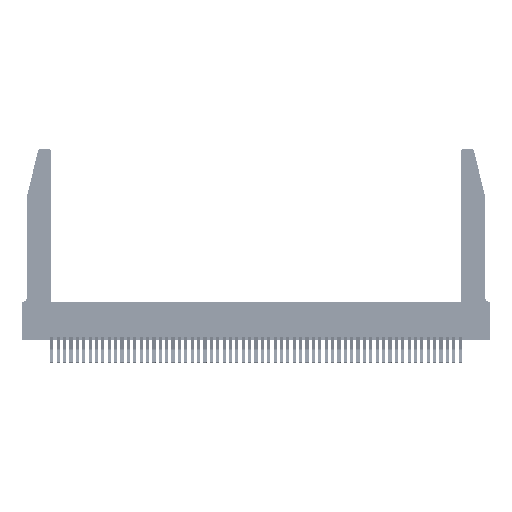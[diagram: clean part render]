
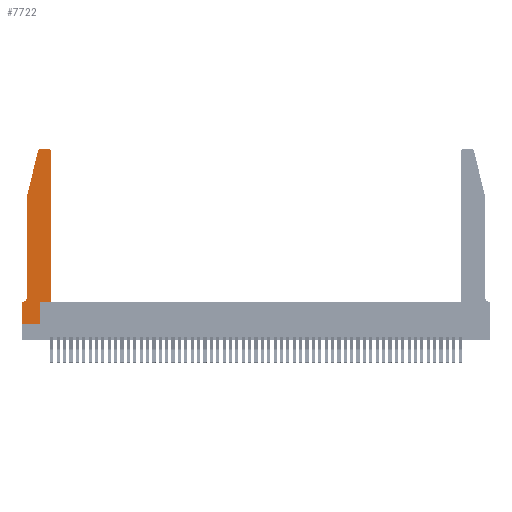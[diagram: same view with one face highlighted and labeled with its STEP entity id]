
A CAD part, top view. The second image highlights one B-rep face of the part: STEP entity #7722.
In plain terms, the highlighted planar face has unit normal (0, 0, 1).
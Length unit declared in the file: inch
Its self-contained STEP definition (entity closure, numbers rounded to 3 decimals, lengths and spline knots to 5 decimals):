
#462 = VERTEX_POINT ( 'NONE', #19016 ) ;
#1192 = VECTOR ( 'NONE', #32694, 39.37008 ) ;
#2263 = CIRCLE ( 'NONE', #45965, 0.03 ) ;
#2456 = VECTOR ( 'NONE', #37878, 39.37008 ) ;
#2739 = DIRECTION ( 'NONE',  ( 0., -1., 0. ) ) ;
#3266 = CARTESIAN_POINT ( 'NONE',  ( 0., 0., 0.37 ) ) ;
#3634 = EDGE_CURVE ( 'NONE', #33077, #462, #50777, .T. ) ;
#3919 = AXIS2_PLACEMENT_3D ( 'NONE', #16741, #32958, #40990 ) ;
#3988 = CARTESIAN_POINT ( 'NONE',  ( 0.0755, 0.35, 0.37 ) ) ;
#4423 = CARTESIAN_POINT ( 'NONE',  ( 0.25487, 2.72718, 0.37 ) ) ;
#4983 = LINE ( 'NONE', #38962, #16243 ) ;
#5503 = EDGE_CURVE ( 'NONE', #47868, #22579, #41599, .T. ) ;
#5510 = ORIENTED_EDGE ( 'NONE', *, *, #7617, .T. ) ;
#6280 = DIRECTION ( 'NONE',  ( 1., 0., 0. ) ) ;
#6669 = CARTESIAN_POINT ( 'NONE',  ( 0., 0.35, 0.37 ) ) ;
#7617 = EDGE_CURVE ( 'NONE', #16330, #10498, #29271, .T. ) ;
#7619 = DIRECTION ( 'NONE',  ( 0., -1., 0. ) ) ;
#7722 = ADVANCED_FACE ( 'NONE', ( #21538 ), #30600, .T. ) ;
#7946 = DIRECTION ( 'NONE',  ( 0., 0., 1. ) ) ;
#8790 = ORIENTED_EDGE ( 'NONE', *, *, #37576, .T. ) ;
#9179 = EDGE_CURVE ( 'NONE', #462, #36047, #2263, .T. ) ;
#9566 = VECTOR ( 'NONE', #16851, 39.37008 ) ;
#10246 = CARTESIAN_POINT ( 'NONE',  ( 0.0055, 0.35, 0.37 ) ) ;
#10498 = VERTEX_POINT ( 'NONE', #32687 ) ;
#10767 = ORIENTED_EDGE ( 'NONE', *, *, #16819, .T. ) ;
#11037 = VERTEX_POINT ( 'NONE', #47966 ) ;
#11060 = ORIENTED_EDGE ( 'NONE', *, *, #3634, .T. ) ;
#11523 = CARTESIAN_POINT ( 'NONE',  ( 0., 0.35, 0.37 ) ) ;
#12094 = EDGE_CURVE ( 'NONE', #36047, #35513, #42078, .T. ) ;
#12353 = EDGE_CURVE ( 'NONE', #41670, #31421, #33108, .T. ) ;
#12401 = ORIENTED_EDGE ( 'NONE', *, *, #9179, .T. ) ;
#12667 = AXIS2_PLACEMENT_3D ( 'NONE', #30721, #14342, #6280 ) ;
#12759 = CARTESIAN_POINT ( 'NONE',  ( 0.0755, 2., 0.37 ) ) ;
#12906 = CARTESIAN_POINT ( 'NONE',  ( 0.4505, 0.35, 0.37 ) ) ;
#14342 = DIRECTION ( 'NONE',  ( 0., 0., 1. ) ) ;
#14795 = ORIENTED_EDGE ( 'NONE', *, *, #12094, .T. ) ;
#16243 = VECTOR ( 'NONE', #31139, 39.37008 ) ;
#16330 = VERTEX_POINT ( 'NONE', #32920 ) ;
#16512 = DIRECTION ( 'NONE',  ( 1., 0., 0. ) ) ;
#16741 = CARTESIAN_POINT ( 'NONE',  ( 0.0055, 0.42, 0.37 ) ) ;
#16819 = EDGE_CURVE ( 'NONE', #31421, #20423, #24379, .T. ) ;
#16851 = DIRECTION ( 'NONE',  ( 1., 0., 0. ) ) ;
#16877 = DIRECTION ( 'NONE',  ( -0.239, -0.971, 0. ) ) ;
#17849 = ORIENTED_EDGE ( 'NONE', *, *, #46955, .T. ) ;
#18648 = DIRECTION ( 'NONE',  ( 1., 0., 0. ) ) ;
#19016 = CARTESIAN_POINT ( 'NONE',  ( 0.4505, 2.72, 0.37 ) ) ;
#19157 = DIRECTION ( 'NONE',  ( -1., 0., 0. ) ) ;
#19419 = CARTESIAN_POINT ( 'NONE',  ( 0.0755, 2., 0.37 ) ) ;
#20423 = VERTEX_POINT ( 'NONE', #3266 ) ;
#20910 = CIRCLE ( 'NONE', #3919, 0.07 ) ;
#21538 = FACE_OUTER_BOUND ( 'NONE', #23923, .T. ) ;
#21671 = LINE ( 'NONE', #19419, #48532 ) ;
#22579 = VERTEX_POINT ( 'NONE', #49021 ) ;
#22969 = CARTESIAN_POINT ( 'NONE',  ( 0.4505, 0.35, 0.37 ) ) ;
#23733 = ORIENTED_EDGE ( 'NONE', *, *, #28901, .T. ) ;
#23749 = VECTOR ( 'NONE', #2739, 39.37008 ) ;
#23923 = EDGE_LOOP ( 'NONE', ( #14795, #17849, #30488, #40120, #23733, #39189, #10767, #8790, #5510, #38531, #11060, #12401 ) ) ;
#24027 = DIRECTION ( 'NONE',  ( 0., 1., 0. ) ) ;
#24379 = LINE ( 'NONE', #47661, #23749 ) ;
#24537 = CARTESIAN_POINT ( 'NONE',  ( 0.4205, 2.72, 0.37 ) ) ;
#25027 = VECTOR ( 'NONE', #16877, 39.37008 ) ;
#26883 = CARTESIAN_POINT ( 'NONE',  ( 0.4205, 2.75, 0.37 ) ) ;
#28901 = EDGE_CURVE ( 'NONE', #11037, #41670, #20910, .T. ) ;
#29271 = LINE ( 'NONE', #34167, #2456 ) ;
#29872 = AXIS2_PLACEMENT_3D ( 'NONE', #6669, #30942, #18648 ) ;
#30488 = ORIENTED_EDGE ( 'NONE', *, *, #5503, .T. ) ;
#30600 = PLANE ( 'NONE',  #29872 ) ;
#30721 = CARTESIAN_POINT ( 'NONE',  ( 0.284, 2.72, 0.37 ) ) ;
#30942 = DIRECTION ( 'NONE',  ( 0., 0., 1. ) ) ;
#31139 = DIRECTION ( 'NONE',  ( 1., 0., 0. ) ) ;
#31213 = VECTOR ( 'NONE', #19157, 39.37008 ) ;
#31421 = VERTEX_POINT ( 'NONE', #11523 ) ;
#32687 = CARTESIAN_POINT ( 'NONE',  ( 0.2865, 0.35, 0.37 ) ) ;
#32694 = DIRECTION ( 'NONE',  ( -1., 0., 0. ) ) ;
#32920 = CARTESIAN_POINT ( 'NONE',  ( 0.2865, 0., 0.37 ) ) ;
#32958 = DIRECTION ( 'NONE',  ( 0., 0., -1. ) ) ;
#33077 = VERTEX_POINT ( 'NONE', #38055 ) ;
#33108 = LINE ( 'NONE', #3988, #1192 ) ;
#34167 = CARTESIAN_POINT ( 'NONE',  ( 0.2865, 0.35, 0.37 ) ) ;
#34839 = VECTOR ( 'NONE', #24027, 39.37008 ) ;
#35513 = VERTEX_POINT ( 'NONE', #43171 ) ;
#36047 = VERTEX_POINT ( 'NONE', #26883 ) ;
#37576 = EDGE_CURVE ( 'NONE', #20423, #16330, #4983, .T. ) ;
#37878 = DIRECTION ( 'NONE',  ( 0., 1., 0. ) ) ;
#38055 = CARTESIAN_POINT ( 'NONE',  ( 0.4505, 0.35, 0.37 ) ) ;
#38531 = ORIENTED_EDGE ( 'NONE', *, *, #48295, .T. ) ;
#38962 = CARTESIAN_POINT ( 'NONE',  ( 0., 0., 0.37 ) ) ;
#39189 = ORIENTED_EDGE ( 'NONE', *, *, #12353, .T. ) ;
#39619 = CIRCLE ( 'NONE', #12667, 0.03 ) ;
#40120 = ORIENTED_EDGE ( 'NONE', *, *, #47699, .T. ) ;
#40990 = DIRECTION ( 'NONE',  ( -1., 0., 0. ) ) ;
#41599 = LINE ( 'NONE', #12759, #25027 ) ;
#41670 = VERTEX_POINT ( 'NONE', #10246 ) ;
#42078 = LINE ( 'NONE', #43263, #31213 ) ;
#43171 = CARTESIAN_POINT ( 'NONE',  ( 0.284, 2.75, 0.37 ) ) ;
#43263 = CARTESIAN_POINT ( 'NONE',  ( 0.2605, 2.75, 0.37 ) ) ;
#45965 = AXIS2_PLACEMENT_3D ( 'NONE', #24537, #7946, #16512 ) ;
#46955 = EDGE_CURVE ( 'NONE', #35513, #47868, #39619, .T. ) ;
#47661 = CARTESIAN_POINT ( 'NONE',  ( 0., 0., 0.37 ) ) ;
#47699 = EDGE_CURVE ( 'NONE', #22579, #11037, #21671, .T. ) ;
#47868 = VERTEX_POINT ( 'NONE', #4423 ) ;
#47966 = CARTESIAN_POINT ( 'NONE',  ( 0.0755, 0.42, 0.37 ) ) ;
#48295 = EDGE_CURVE ( 'NONE', #10498, #33077, #50346, .T. ) ;
#48532 = VECTOR ( 'NONE', #7619, 39.37008 ) ;
#49021 = CARTESIAN_POINT ( 'NONE',  ( 0.0755, 2., 0.37 ) ) ;
#50346 = LINE ( 'NONE', #12906, #9566 ) ;
#50777 = LINE ( 'NONE', #22969, #34839 ) ;
